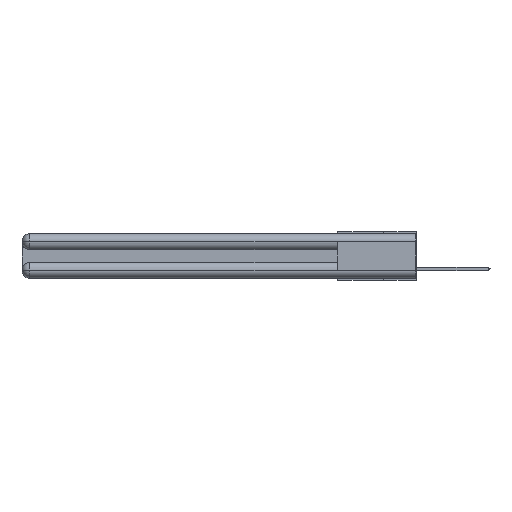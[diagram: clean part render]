
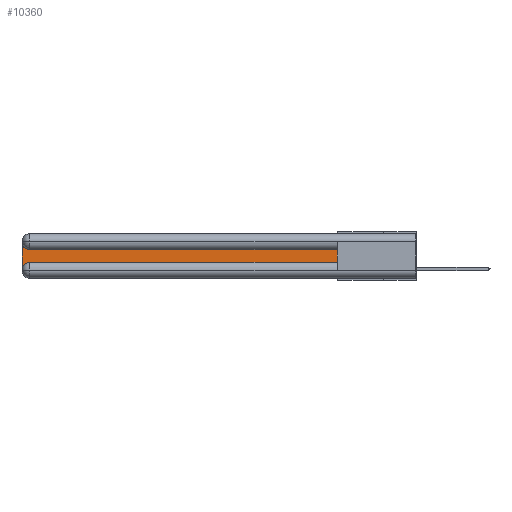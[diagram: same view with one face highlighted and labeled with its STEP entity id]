
A CAD part, left-side view. The second image highlights one B-rep face of the part: STEP entity #10360.
In plain terms, the highlighted planar face has unit normal (-1, 0, 0).
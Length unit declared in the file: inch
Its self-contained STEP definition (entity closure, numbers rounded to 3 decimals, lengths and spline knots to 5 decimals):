
#25 = LINE ( 'NONE', #23313, #9321 ) ;
#108 = EDGE_CURVE ( 'NONE', #7816, #10239, #25077, .T. ) ;
#246 = VERTEX_POINT ( 'NONE', #25742 ) ;
#985 = EDGE_CURVE ( 'NONE', #3883, #246, #12221, .T. ) ;
#1367 = DIRECTION ( 'NONE',  ( 1., 0., 0. ) ) ;
#2624 = DIRECTION ( 'NONE',  ( 1., 0., 0. ) ) ;
#3883 = VERTEX_POINT ( 'NONE', #6069 ) ;
#4012 = AXIS2_PLACEMENT_3D ( 'NONE', #13814, #2624, #25242 ) ;
#4058 = EDGE_CURVE ( 'NONE', #246, #14654, #25, .T. ) ;
#4134 = LINE ( 'NONE', #11616, #5548 ) ;
#5548 = VECTOR ( 'NONE', #11330, 39.37008 ) ;
#6069 = CARTESIAN_POINT ( 'NONE',  ( 0.075, 2.94, -0.2175 ) ) ;
#6561 = ORIENTED_EDGE ( 'NONE', *, *, #18617, .T. ) ;
#7657 = ORIENTED_EDGE ( 'NONE', *, *, #4058, .T. ) ;
#7816 = VERTEX_POINT ( 'NONE', #13383 ) ;
#9224 = CARTESIAN_POINT ( 'NONE',  ( 0.075, 0.6, -0.2175 ) ) ;
#9248 = VERTEX_POINT ( 'NONE', #24794 ) ;
#9284 = CARTESIAN_POINT ( 'NONE',  ( 0.075, 3., -0.0625 ) ) ;
#9321 = VECTOR ( 'NONE', #13920, 39.37008 ) ;
#10239 = VERTEX_POINT ( 'NONE', #9284 ) ;
#10360 = ADVANCED_FACE ( 'NONE', ( #13836 ), #12691, .F. ) ;
#10787 = CARTESIAN_POINT ( 'NONE',  ( 0.075, 3., -0.2175 ) ) ;
#11043 = ORIENTED_EDGE ( 'NONE', *, *, #108, .T. ) ;
#11330 = DIRECTION ( 'NONE',  ( 0., 1., 0. ) ) ;
#11616 = CARTESIAN_POINT ( 'NONE',  ( 0.075, 0.6, -0.1225 ) ) ;
#12221 = LINE ( 'NONE', #9224, #15416 ) ;
#12691 = PLANE ( 'NONE',  #29384 ) ;
#13178 = CARTESIAN_POINT ( 'NONE',  ( 0.075, 0.6, -0.1225 ) ) ;
#13383 = CARTESIAN_POINT ( 'NONE',  ( 0.075, 2.94, -0.1225 ) ) ;
#13814 = CARTESIAN_POINT ( 'NONE',  ( 0.075, 2.94, -0.0625 ) ) ;
#13836 = FACE_OUTER_BOUND ( 'NONE', #17930, .T. ) ;
#13920 = DIRECTION ( 'NONE',  ( 0., 0., 1. ) ) ;
#14654 = VERTEX_POINT ( 'NONE', #13178 ) ;
#15416 = VECTOR ( 'NONE', #27448, 39.37008 ) ;
#17162 = DIRECTION ( 'NONE',  ( 0., 0., -1. ) ) ;
#17872 = DIRECTION ( 'NONE',  ( 0., 0., -1. ) ) ;
#17930 = EDGE_LOOP ( 'NONE', ( #28673, #11043, #25634, #6561, #27009, #7657 ) ) ;
#18617 = EDGE_CURVE ( 'NONE', #9248, #3883, #24707, .T. ) ;
#18823 = DIRECTION ( 'NONE',  ( 0., 0., -1. ) ) ;
#21177 = EDGE_CURVE ( 'NONE', #10239, #9248, #24660, .T. ) ;
#21468 = CARTESIAN_POINT ( 'NONE',  ( 0.075, 3., -0.1225 ) ) ;
#21485 = VECTOR ( 'NONE', #17872, 39.37008 ) ;
#23313 = CARTESIAN_POINT ( 'NONE',  ( 0.075, 0.6, -0.2175 ) ) ;
#23734 = AXIS2_PLACEMENT_3D ( 'NONE', #26072, #28370, #18823 ) ;
#24660 = LINE ( 'NONE', #10787, #21485 ) ;
#24707 = CIRCLE ( 'NONE', #23734, 0.06 ) ;
#24794 = CARTESIAN_POINT ( 'NONE',  ( 0.075, 3., -0.2775 ) ) ;
#25077 = CIRCLE ( 'NONE', #4012, 0.06 ) ;
#25242 = DIRECTION ( 'NONE',  ( 0., 0., -1. ) ) ;
#25308 = EDGE_CURVE ( 'NONE', #14654, #7816, #4134, .T. ) ;
#25634 = ORIENTED_EDGE ( 'NONE', *, *, #21177, .T. ) ;
#25742 = CARTESIAN_POINT ( 'NONE',  ( 0.075, 0.6, -0.2175 ) ) ;
#26072 = CARTESIAN_POINT ( 'NONE',  ( 0.075, 2.94, -0.2775 ) ) ;
#27009 = ORIENTED_EDGE ( 'NONE', *, *, #985, .T. ) ;
#27448 = DIRECTION ( 'NONE',  ( 0., -1., 0. ) ) ;
#28370 = DIRECTION ( 'NONE',  ( 1., 0., 0. ) ) ;
#28673 = ORIENTED_EDGE ( 'NONE', *, *, #25308, .T. ) ;
#29384 = AXIS2_PLACEMENT_3D ( 'NONE', #21468, #1367, #17162 ) ;
